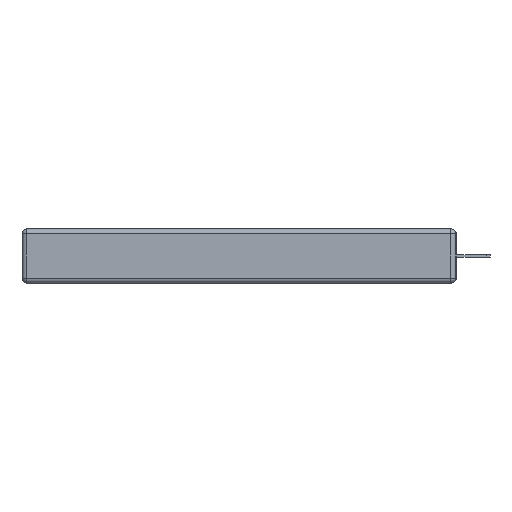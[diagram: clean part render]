
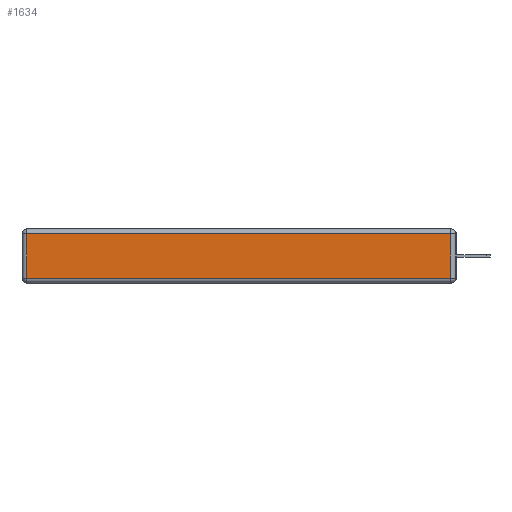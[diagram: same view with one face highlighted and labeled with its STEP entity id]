
A CAD part, left-side view. The second image highlights one B-rep face of the part: STEP entity #1634.
In plain terms, the highlighted planar face has unit normal (-1, 0, 0).
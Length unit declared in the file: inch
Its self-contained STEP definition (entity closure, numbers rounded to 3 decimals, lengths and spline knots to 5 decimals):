
#1068 = DIRECTION ( 'NONE',  ( 0., 1., 0. ) ) ;
#1495 = DIRECTION ( 'NONE',  ( -1., 0., 0. ) ) ;
#1566 = VECTOR ( 'NONE', #3860, 39.37008 ) ;
#1634 = ADVANCED_FACE ( 'NONE', ( #4079 ), #9297, .T. ) ;
#2057 = VECTOR ( 'NONE', #7573, 39.37008 ) ;
#3539 = CARTESIAN_POINT ( 'NONE',  ( 0., 0.03, -0.313 ) ) ;
#3773 = LINE ( 'NONE', #14395, #1566 ) ;
#3860 = DIRECTION ( 'NONE',  ( 0., -1., 0. ) ) ;
#3887 = CARTESIAN_POINT ( 'NONE',  ( 0., 0.03, -0.343 ) ) ;
#4078 = VERTEX_POINT ( 'NONE', #15446 ) ;
#4079 = FACE_OUTER_BOUND ( 'NONE', #9646, .T. ) ;
#4349 = DIRECTION ( 'NONE',  ( 0., 0., -1. ) ) ;
#4545 = LINE ( 'NONE', #9767, #7836 ) ;
#5122 = CARTESIAN_POINT ( 'NONE',  ( 0., 0.03, -0.03 ) ) ;
#5536 = DIRECTION ( 'NONE',  ( 0., 0., 1. ) ) ;
#6032 = LINE ( 'NONE', #11342, #10199 ) ;
#7573 = DIRECTION ( 'NONE',  ( 0., 0., 1. ) ) ;
#7811 = ORIENTED_EDGE ( 'NONE', *, *, #16475, .T. ) ;
#7836 = VECTOR ( 'NONE', #1068, 39.37008 ) ;
#7891 = VERTEX_POINT ( 'NONE', #3539 ) ;
#8309 = AXIS2_PLACEMENT_3D ( 'NONE', #14533, #1495, #5536 ) ;
#9017 = VERTEX_POINT ( 'NONE', #9883 ) ;
#9085 = EDGE_CURVE ( 'NONE', #7891, #10010, #11994, .T. ) ;
#9297 = PLANE ( 'NONE',  #8309 ) ;
#9646 = EDGE_LOOP ( 'NONE', ( #10341, #10605, #14382, #7811 ) ) ;
#9767 = CARTESIAN_POINT ( 'NONE',  ( 0., 2.75, -0.03 ) ) ;
#9883 = CARTESIAN_POINT ( 'NONE',  ( 0., 2.72, -0.03 ) ) ;
#10010 = VERTEX_POINT ( 'NONE', #5122 ) ;
#10199 = VECTOR ( 'NONE', #4349, 39.37008 ) ;
#10341 = ORIENTED_EDGE ( 'NONE', *, *, #12822, .T. ) ;
#10605 = ORIENTED_EDGE ( 'NONE', *, *, #9085, .T. ) ;
#11100 = EDGE_CURVE ( 'NONE', #10010, #9017, #4545, .T. ) ;
#11342 = CARTESIAN_POINT ( 'NONE',  ( 0., 2.72, -0.343 ) ) ;
#11994 = LINE ( 'NONE', #3887, #2057 ) ;
#12822 = EDGE_CURVE ( 'NONE', #4078, #7891, #3773, .T. ) ;
#14382 = ORIENTED_EDGE ( 'NONE', *, *, #11100, .T. ) ;
#14395 = CARTESIAN_POINT ( 'NONE',  ( 0., 0., -0.313 ) ) ;
#14533 = CARTESIAN_POINT ( 'NONE',  ( 0., 0., -0.343 ) ) ;
#15446 = CARTESIAN_POINT ( 'NONE',  ( 0., 2.72, -0.313 ) ) ;
#16475 = EDGE_CURVE ( 'NONE', #9017, #4078, #6032, .T. ) ;
